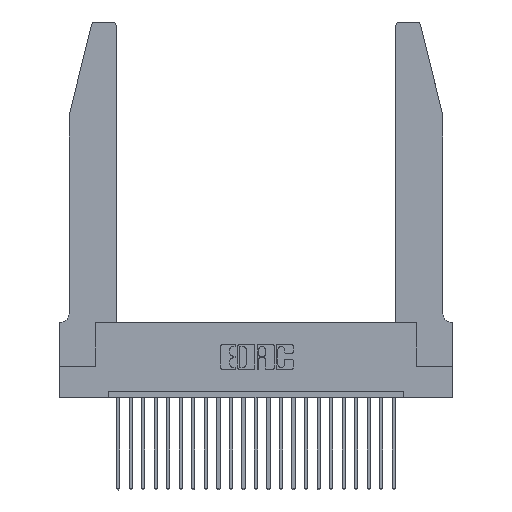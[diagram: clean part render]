
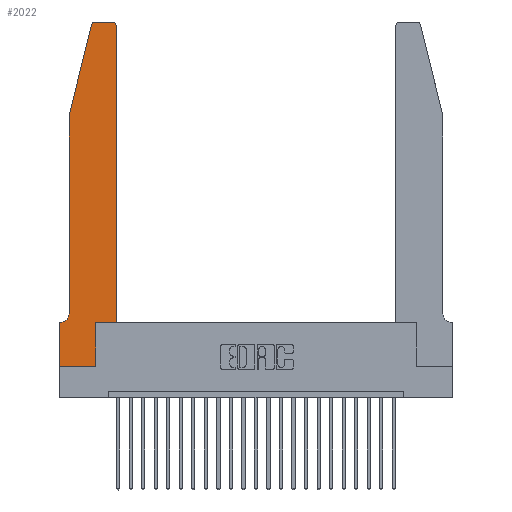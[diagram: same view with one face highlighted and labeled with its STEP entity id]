
A CAD part, top view. The second image highlights one B-rep face of the part: STEP entity #2022.
In plain terms, the highlighted planar face has unit normal (0, 0, 1).
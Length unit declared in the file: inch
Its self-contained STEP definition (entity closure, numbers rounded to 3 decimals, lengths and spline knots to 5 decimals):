
#274 = VERTEX_POINT ( 'NONE', #21954 ) ;
#278 = DIRECTION ( 'NONE',  ( 1., 0., 0. ) ) ;
#293 = CARTESIAN_POINT ( 'NONE',  ( 0.4205, 2.75, 0.37 ) ) ;
#573 = CARTESIAN_POINT ( 'NONE',  ( 0.25487, 2.72718, 0.37 ) ) ;
#701 = EDGE_CURVE ( 'NONE', #5016, #6302, #1194, .T. ) ;
#1194 = LINE ( 'NONE', #19525, #10716 ) ;
#1259 = LINE ( 'NONE', #22319, #13142 ) ;
#1464 = DIRECTION ( 'NONE',  ( 0., 1., 0. ) ) ;
#1739 = LINE ( 'NONE', #6841, #15070 ) ;
#2022 = ADVANCED_FACE ( 'NONE', ( #10954 ), #11601, .T. ) ;
#2146 = CARTESIAN_POINT ( 'NONE',  ( 0., 0.35, 0.37 ) ) ;
#2456 = EDGE_CURVE ( 'NONE', #16398, #23324, #2592, .T. ) ;
#2592 = LINE ( 'NONE', #16936, #19875 ) ;
#2892 = EDGE_CURVE ( 'NONE', #15912, #8772, #15649, .T. ) ;
#3551 = CARTESIAN_POINT ( 'NONE',  ( 0.0755, 0.42, 0.37 ) ) ;
#3604 = CIRCLE ( 'NONE', #13738, 0.03 ) ;
#4027 = EDGE_CURVE ( 'NONE', #13759, #5016, #9936, .T. ) ;
#4573 = DIRECTION ( 'NONE',  ( 0., 1., 0. ) ) ;
#4809 = DIRECTION ( 'NONE',  ( 0., -1., 0. ) ) ;
#5016 = VERTEX_POINT ( 'NONE', #22436 ) ;
#5236 = ORIENTED_EDGE ( 'NONE', *, *, #2892, .T. ) ;
#5432 = EDGE_CURVE ( 'NONE', #274, #13759, #1739, .T. ) ;
#5617 = LINE ( 'NONE', #23784, #22883 ) ;
#5750 = CARTESIAN_POINT ( 'NONE',  ( 0.0755, 2., 0.37 ) ) ;
#6302 = VERTEX_POINT ( 'NONE', #13990 ) ;
#6784 = VERTEX_POINT ( 'NONE', #3551 ) ;
#6841 = CARTESIAN_POINT ( 'NONE',  ( 0.2865, 0.35, 0.37 ) ) ;
#7268 = EDGE_LOOP ( 'NONE', ( #10811, #13750, #5236, #22773, #11393, #8706, #13254, #8723, #24119, #21620, #18248, #7539 ) ) ;
#7300 = EDGE_CURVE ( 'NONE', #10098, #15912, #10913, .T. ) ;
#7334 = CARTESIAN_POINT ( 'NONE',  ( 0., 0., 0.37 ) ) ;
#7539 = ORIENTED_EDGE ( 'NONE', *, *, #9682, .T. ) ;
#7825 = CARTESIAN_POINT ( 'NONE',  ( 0.2605, 2.75, 0.37 ) ) ;
#7854 = VECTOR ( 'NONE', #278, 39.37008 ) ;
#7879 = VERTEX_POINT ( 'NONE', #293 ) ;
#8706 = ORIENTED_EDGE ( 'NONE', *, *, #20359, .T. ) ;
#8723 = ORIENTED_EDGE ( 'NONE', *, *, #16358, .T. ) ;
#8772 = VERTEX_POINT ( 'NONE', #20319 ) ;
#9682 = EDGE_CURVE ( 'NONE', #6302, #7879, #3604, .T. ) ;
#9876 = LINE ( 'NONE', #7825, #14355 ) ;
#9936 = LINE ( 'NONE', #15314, #7854 ) ;
#9972 = CARTESIAN_POINT ( 'NONE',  ( 0.284, 2.75, 0.37 ) ) ;
#10021 = DIRECTION ( 'NONE',  ( 1., 0., 0. ) ) ;
#10098 = VERTEX_POINT ( 'NONE', #9972 ) ;
#10716 = VECTOR ( 'NONE', #1464, 39.37008 ) ;
#10811 = ORIENTED_EDGE ( 'NONE', *, *, #24551, .T. ) ;
#10913 = CIRCLE ( 'NONE', #18878, 0.03 ) ;
#10954 = FACE_OUTER_BOUND ( 'NONE', #7268, .T. ) ;
#11153 = CARTESIAN_POINT ( 'NONE',  ( 0., 0.35, 0.37 ) ) ;
#11393 = ORIENTED_EDGE ( 'NONE', *, *, #12080, .T. ) ;
#11494 = DIRECTION ( 'NONE',  ( 0., -1., 0. ) ) ;
#11601 = PLANE ( 'NONE',  #20094 ) ;
#11754 = CIRCLE ( 'NONE', #13770, 0.07 ) ;
#12080 = EDGE_CURVE ( 'NONE', #6784, #15001, #11754, .T. ) ;
#12346 = DIRECTION ( 'NONE',  ( 1., 0., 0. ) ) ;
#12398 = CARTESIAN_POINT ( 'NONE',  ( 0.0055, 0.42, 0.37 ) ) ;
#13142 = VECTOR ( 'NONE', #17208, 39.37008 ) ;
#13254 = ORIENTED_EDGE ( 'NONE', *, *, #2456, .T. ) ;
#13738 = AXIS2_PLACEMENT_3D ( 'NONE', #18206, #14499, #18466 ) ;
#13750 = ORIENTED_EDGE ( 'NONE', *, *, #7300, .T. ) ;
#13759 = VERTEX_POINT ( 'NONE', #16488 ) ;
#13770 = AXIS2_PLACEMENT_3D ( 'NONE', #12398, #18168, #22005 ) ;
#13817 = CARTESIAN_POINT ( 'NONE',  ( 0.0055, 0.35, 0.37 ) ) ;
#13990 = CARTESIAN_POINT ( 'NONE',  ( 0.4505, 2.72, 0.37 ) ) ;
#14355 = VECTOR ( 'NONE', #23136, 39.37008 ) ;
#14499 = DIRECTION ( 'NONE',  ( 0., 0., 1. ) ) ;
#14557 = LINE ( 'NONE', #7334, #15437 ) ;
#15001 = VERTEX_POINT ( 'NONE', #13817 ) ;
#15070 = VECTOR ( 'NONE', #4573, 39.37008 ) ;
#15314 = CARTESIAN_POINT ( 'NONE',  ( 0.4505, 0.35, 0.37 ) ) ;
#15437 = VECTOR ( 'NONE', #20824, 39.37008 ) ;
#15649 = LINE ( 'NONE', #5750, #16292 ) ;
#15912 = VERTEX_POINT ( 'NONE', #573 ) ;
#16292 = VECTOR ( 'NONE', #21145, 39.37008 ) ;
#16358 = EDGE_CURVE ( 'NONE', #23324, #274, #14557, .T. ) ;
#16398 = VERTEX_POINT ( 'NONE', #11153 ) ;
#16488 = CARTESIAN_POINT ( 'NONE',  ( 0.2865, 0.35, 0.37 ) ) ;
#16936 = CARTESIAN_POINT ( 'NONE',  ( 0., 0., 0.37 ) ) ;
#17208 = DIRECTION ( 'NONE',  ( -1., 0., 0. ) ) ;
#18168 = DIRECTION ( 'NONE',  ( 0., 0., -1. ) ) ;
#18206 = CARTESIAN_POINT ( 'NONE',  ( 0.4205, 2.72, 0.37 ) ) ;
#18248 = ORIENTED_EDGE ( 'NONE', *, *, #701, .T. ) ;
#18466 = DIRECTION ( 'NONE',  ( 1., 0., 0. ) ) ;
#18878 = AXIS2_PLACEMENT_3D ( 'NONE', #23751, #23916, #12346 ) ;
#19525 = CARTESIAN_POINT ( 'NONE',  ( 0.4505, 0.35, 0.37 ) ) ;
#19875 = VECTOR ( 'NONE', #11494, 39.37008 ) ;
#20094 = AXIS2_PLACEMENT_3D ( 'NONE', #2146, #21722, #10021 ) ;
#20319 = CARTESIAN_POINT ( 'NONE',  ( 0.0755, 2., 0.37 ) ) ;
#20359 = EDGE_CURVE ( 'NONE', #15001, #16398, #1259, .T. ) ;
#20824 = DIRECTION ( 'NONE',  ( 1., 0., 0. ) ) ;
#21145 = DIRECTION ( 'NONE',  ( -0.239, -0.971, 0. ) ) ;
#21620 = ORIENTED_EDGE ( 'NONE', *, *, #4027, .T. ) ;
#21722 = DIRECTION ( 'NONE',  ( 0., 0., 1. ) ) ;
#21954 = CARTESIAN_POINT ( 'NONE',  ( 0.2865, 0., 0.37 ) ) ;
#22005 = DIRECTION ( 'NONE',  ( -1., 0., 0. ) ) ;
#22319 = CARTESIAN_POINT ( 'NONE',  ( 0.0755, 0.35, 0.37 ) ) ;
#22436 = CARTESIAN_POINT ( 'NONE',  ( 0.4505, 0.35, 0.37 ) ) ;
#22439 = EDGE_CURVE ( 'NONE', #8772, #6784, #5617, .T. ) ;
#22773 = ORIENTED_EDGE ( 'NONE', *, *, #22439, .T. ) ;
#22883 = VECTOR ( 'NONE', #4809, 39.37008 ) ;
#23136 = DIRECTION ( 'NONE',  ( -1., 0., 0. ) ) ;
#23324 = VERTEX_POINT ( 'NONE', #24047 ) ;
#23751 = CARTESIAN_POINT ( 'NONE',  ( 0.284, 2.72, 0.37 ) ) ;
#23784 = CARTESIAN_POINT ( 'NONE',  ( 0.0755, 2., 0.37 ) ) ;
#23916 = DIRECTION ( 'NONE',  ( 0., 0., 1. ) ) ;
#24047 = CARTESIAN_POINT ( 'NONE',  ( 0., 0., 0.37 ) ) ;
#24119 = ORIENTED_EDGE ( 'NONE', *, *, #5432, .T. ) ;
#24551 = EDGE_CURVE ( 'NONE', #7879, #10098, #9876, .T. ) ;
